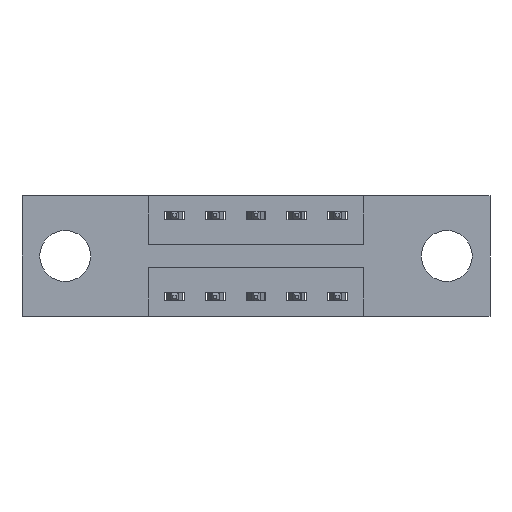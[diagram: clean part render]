
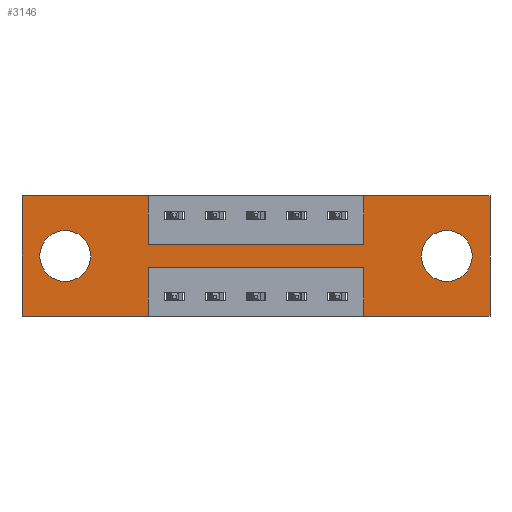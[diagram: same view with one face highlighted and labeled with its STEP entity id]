
A CAD part, front view. The second image highlights one B-rep face of the part: STEP entity #3146.
In plain terms, the highlighted planar face has unit normal (0, -1, 0).
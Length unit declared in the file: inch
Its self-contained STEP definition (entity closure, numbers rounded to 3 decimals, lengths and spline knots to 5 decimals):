
#69 = EDGE_CURVE ( 'NONE', #6793, #6067, #6084, .T. ) ;
#86 = EDGE_CURVE ( 'NONE', #6093, #6793, #6535, .T. ) ;
#127 = EDGE_CURVE ( 'NONE', #1687, #6093, #5450, .T. ) ;
#129 = CARTESIAN_POINT ( 'NONE',  ( 0.1325, 0., -0.185 ) ) ;
#203 = EDGE_CURVE ( 'NONE', #4125, #7672, #4257, .T. ) ;
#245 = CARTESIAN_POINT ( 'NONE',  ( 0.1325, 0., -0.263 ) ) ;
#272 = CARTESIAN_POINT ( 'NONE',  ( 0.3875, 0., 0. ) ) ;
#301 = VECTOR ( 'NONE', #5108, 39.37008 ) ;
#306 = DIRECTION ( 'NONE',  ( 0., 0., -1. ) ) ;
#368 = AXIS2_PLACEMENT_3D ( 'NONE', #5971, #5891, #1050 ) ;
#425 = CARTESIAN_POINT ( 'NONE',  ( 0.3875, 0., -0.37 ) ) ;
#450 = DIRECTION ( 'NONE',  ( 0., 0., -1. ) ) ;
#490 = CARTESIAN_POINT ( 'NONE',  ( 0.3875, 0., -0.15 ) ) ;
#520 = VECTOR ( 'NONE', #5414, 39.37008 ) ;
#553 = VERTEX_POINT ( 'NONE', #5676 ) ;
#614 = DIRECTION ( 'NONE',  ( 0., 0., 1. ) ) ;
#622 = CARTESIAN_POINT ( 'NONE',  ( 1.0475, 0., 0. ) ) ;
#652 = LINE ( 'NONE', #5789, #520 ) ;
#660 = EDGE_LOOP ( 'NONE', ( #7352, #1690, #7847, #6257, #4258, #1886, #1897, #4024, #5844, #7938, #4733, #712 ) ) ;
#696 = DIRECTION ( 'NONE',  ( 1., 0., 0. ) ) ;
#712 = ORIENTED_EDGE ( 'NONE', *, *, #5054, .F. ) ;
#835 = DIRECTION ( 'NONE',  ( 0., 0., -1. ) ) ;
#959 = DIRECTION ( 'NONE',  ( 0., 0., -1. ) ) ;
#968 = DIRECTION ( 'NONE',  ( 0., 1., 0. ) ) ;
#970 = CARTESIAN_POINT ( 'NONE',  ( 1.3025, 0., -0.185 ) ) ;
#979 = EDGE_CURVE ( 'NONE', #4657, #2655, #5480, .T. ) ;
#984 = EDGE_LOOP ( 'NONE', ( #4315, #3857 ) ) ;
#1050 = DIRECTION ( 'NONE',  ( 0., 0., -1. ) ) ;
#1095 = DIRECTION ( 'NONE',  ( 0., -1., 0. ) ) ;
#1530 = CIRCLE ( 'NONE', #3307, 0.078 ) ;
#1537 = VECTOR ( 'NONE', #450, 39.37008 ) ;
#1547 = LINE ( 'NONE', #425, #1537 ) ;
#1555 = EDGE_LOOP ( 'NONE', ( #2688, #7342 ) ) ;
#1558 = PLANE ( 'NONE',  #1777 ) ;
#1678 = VERTEX_POINT ( 'NONE', #3285 ) ;
#1687 = VERTEX_POINT ( 'NONE', #7633 ) ;
#1690 = ORIENTED_EDGE ( 'NONE', *, *, #7239, .F. ) ;
#1777 = AXIS2_PLACEMENT_3D ( 'NONE', #2217, #1095, #835 ) ;
#1886 = ORIENTED_EDGE ( 'NONE', *, *, #6462, .F. ) ;
#1897 = ORIENTED_EDGE ( 'NONE', *, *, #69, .F. ) ;
#1908 = VECTOR ( 'NONE', #5339, 39.37008 ) ;
#1909 = CARTESIAN_POINT ( 'NONE',  ( 1.3025, 0., -0.107 ) ) ;
#2067 = CARTESIAN_POINT ( 'NONE',  ( 1.435, 0., 0. ) ) ;
#2141 = VERTEX_POINT ( 'NONE', #8088 ) ;
#2177 = CARTESIAN_POINT ( 'NONE',  ( 1.435, 0., -0.37 ) ) ;
#2215 = EDGE_CURVE ( 'NONE', #2897, #1687, #2709, .T. ) ;
#2217 = CARTESIAN_POINT ( 'NONE',  ( 0., 0., -0.37 ) ) ;
#2349 = CARTESIAN_POINT ( 'NONE',  ( 0., 0., 0. ) ) ;
#2655 = VERTEX_POINT ( 'NONE', #2177 ) ;
#2688 = ORIENTED_EDGE ( 'NONE', *, *, #7082, .T. ) ;
#2709 = LINE ( 'NONE', #7521, #1908 ) ;
#2889 = EDGE_CURVE ( 'NONE', #2655, #2141, #5843, .T. ) ;
#2897 = VERTEX_POINT ( 'NONE', #2349 ) ;
#2913 = VERTEX_POINT ( 'NONE', #3804 ) ;
#2995 = CARTESIAN_POINT ( 'NONE',  ( 0., 0., 0. ) ) ;
#3004 = CARTESIAN_POINT ( 'NONE',  ( 1.435, 0., 0. ) ) ;
#3022 = CIRCLE ( 'NONE', #5811, 0.078 ) ;
#3045 = LINE ( 'NONE', #5154, #301 ) ;
#3075 = DIRECTION ( 'NONE',  ( 0., 0., 1. ) ) ;
#3105 = CARTESIAN_POINT ( 'NONE',  ( 1.0475, 0., -0.15 ) ) ;
#3142 = DIRECTION ( 'NONE',  ( -1., 0., 0. ) ) ;
#3146 = ADVANCED_FACE ( 'NONE', ( #5112, #7832, #4437 ), #1558, .T. ) ;
#3285 = CARTESIAN_POINT ( 'NONE',  ( 0.3875, 0., -0.22 ) ) ;
#3297 = EDGE_CURVE ( 'NONE', #4841, #2897, #7141, .T. ) ;
#3307 = AXIS2_PLACEMENT_3D ( 'NONE', #129, #8227, #8140 ) ;
#3403 = CARTESIAN_POINT ( 'NONE',  ( 0.1325, 0., -0.185 ) ) ;
#3646 = CARTESIAN_POINT ( 'NONE',  ( 0.1325, 0., -0.107 ) ) ;
#3804 = CARTESIAN_POINT ( 'NONE',  ( 1.0475, 0., -0.22 ) ) ;
#3857 = ORIENTED_EDGE ( 'NONE', *, *, #203, .T. ) ;
#3920 = CARTESIAN_POINT ( 'NONE',  ( 0.3875, 0., -0.37 ) ) ;
#4024 = ORIENTED_EDGE ( 'NONE', *, *, #86, .F. ) ;
#4125 = VERTEX_POINT ( 'NONE', #245 ) ;
#4225 = DIRECTION ( 'NONE',  ( 0., 0., -1. ) ) ;
#4257 = CIRCLE ( 'NONE', #4466, 0.078 ) ;
#4258 = ORIENTED_EDGE ( 'NONE', *, *, #979, .F. ) ;
#4315 = ORIENTED_EDGE ( 'NONE', *, *, #7189, .T. ) ;
#4417 = VECTOR ( 'NONE', #3142, 39.37008 ) ;
#4437 = FACE_OUTER_BOUND ( 'NONE', #660, .T. ) ;
#4466 = AXIS2_PLACEMENT_3D ( 'NONE', #3403, #8249, #5424 ) ;
#4657 = VERTEX_POINT ( 'NONE', #3004 ) ;
#4733 = ORIENTED_EDGE ( 'NONE', *, *, #3297, .F. ) ;
#4841 = VERTEX_POINT ( 'NONE', #7290 ) ;
#4845 = EDGE_CURVE ( 'NONE', #553, #5308, #6419, .T. ) ;
#5046 = VECTOR ( 'NONE', #306, 39.37008 ) ;
#5054 = EDGE_CURVE ( 'NONE', #5716, #4841, #6708, .T. ) ;
#5108 = DIRECTION ( 'NONE',  ( 1., 0., 0. ) ) ;
#5112 = FACE_BOUND ( 'NONE', #1555, .T. ) ;
#5154 = CARTESIAN_POINT ( 'NONE',  ( 0., 0., 0. ) ) ;
#5299 = VECTOR ( 'NONE', #4225, 39.37008 ) ;
#5308 = VERTEX_POINT ( 'NONE', #1909 ) ;
#5339 = DIRECTION ( 'NONE',  ( 1., 0., 0. ) ) ;
#5369 = VECTOR ( 'NONE', #8234, 39.37008 ) ;
#5413 = LINE ( 'NONE', #8226, #5369 ) ;
#5414 = DIRECTION ( 'NONE',  ( -1., 0., 0. ) ) ;
#5424 = DIRECTION ( 'NONE',  ( 0., 0., 1. ) ) ;
#5450 = LINE ( 'NONE', #272, #5046 ) ;
#5480 = LINE ( 'NONE', #2067, #5299 ) ;
#5541 = DIRECTION ( 'NONE',  ( -1., 0., 0. ) ) ;
#5676 = CARTESIAN_POINT ( 'NONE',  ( 1.3025, 0., -0.263 ) ) ;
#5716 = VERTEX_POINT ( 'NONE', #3920 ) ;
#5789 = CARTESIAN_POINT ( 'NONE',  ( 0.3875, 0., -0.22 ) ) ;
#5811 = AXIS2_PLACEMENT_3D ( 'NONE', #970, #968, #959 ) ;
#5843 = LINE ( 'NONE', #6391, #4417 ) ;
#5844 = ORIENTED_EDGE ( 'NONE', *, *, #127, .F. ) ;
#5891 = DIRECTION ( 'NONE',  ( 0., 1., 0. ) ) ;
#5971 = CARTESIAN_POINT ( 'NONE',  ( 1.3025, 0., -0.185 ) ) ;
#6067 = VERTEX_POINT ( 'NONE', #7946 ) ;
#6084 = LINE ( 'NONE', #622, #6367 ) ;
#6087 = VECTOR ( 'NONE', #3075, 39.37008 ) ;
#6093 = VERTEX_POINT ( 'NONE', #7624 ) ;
#6178 = VECTOR ( 'NONE', #696, 39.37008 ) ;
#6257 = ORIENTED_EDGE ( 'NONE', *, *, #2889, .F. ) ;
#6284 = CARTESIAN_POINT ( 'NONE',  ( 0., 0., -0.37 ) ) ;
#6367 = VECTOR ( 'NONE', #614, 39.37008 ) ;
#6391 = CARTESIAN_POINT ( 'NONE',  ( 0., 0., -0.37 ) ) ;
#6419 = CIRCLE ( 'NONE', #368, 0.078 ) ;
#6462 = EDGE_CURVE ( 'NONE', #6067, #4657, #3045, .T. ) ;
#6535 = LINE ( 'NONE', #490, #6178 ) ;
#6685 = VECTOR ( 'NONE', #5541, 39.37008 ) ;
#6708 = LINE ( 'NONE', #6284, #6685 ) ;
#6793 = VERTEX_POINT ( 'NONE', #3105 ) ;
#7082 = EDGE_CURVE ( 'NONE', #5308, #553, #3022, .T. ) ;
#7140 = EDGE_CURVE ( 'NONE', #1678, #5716, #1547, .T. ) ;
#7141 = LINE ( 'NONE', #2995, #6087 ) ;
#7189 = EDGE_CURVE ( 'NONE', #7672, #4125, #1530, .T. ) ;
#7239 = EDGE_CURVE ( 'NONE', #2913, #1678, #652, .T. ) ;
#7290 = CARTESIAN_POINT ( 'NONE',  ( 0., 0., -0.37 ) ) ;
#7342 = ORIENTED_EDGE ( 'NONE', *, *, #4845, .T. ) ;
#7352 = ORIENTED_EDGE ( 'NONE', *, *, #7140, .F. ) ;
#7521 = CARTESIAN_POINT ( 'NONE',  ( 0., 0., 0. ) ) ;
#7624 = CARTESIAN_POINT ( 'NONE',  ( 0.3875, 0., -0.15 ) ) ;
#7633 = CARTESIAN_POINT ( 'NONE',  ( 0.3875, 0., 0. ) ) ;
#7672 = VERTEX_POINT ( 'NONE', #3646 ) ;
#7832 = FACE_BOUND ( 'NONE', #984, .T. ) ;
#7847 = ORIENTED_EDGE ( 'NONE', *, *, #7892, .F. ) ;
#7892 = EDGE_CURVE ( 'NONE', #2141, #2913, #5413, .T. ) ;
#7938 = ORIENTED_EDGE ( 'NONE', *, *, #2215, .F. ) ;
#7946 = CARTESIAN_POINT ( 'NONE',  ( 1.0475, 0., 0. ) ) ;
#8088 = CARTESIAN_POINT ( 'NONE',  ( 1.0475, 0., -0.37 ) ) ;
#8140 = DIRECTION ( 'NONE',  ( 0., 0., 1. ) ) ;
#8226 = CARTESIAN_POINT ( 'NONE',  ( 1.0475, 0., -0.37 ) ) ;
#8227 = DIRECTION ( 'NONE',  ( 0., 1., 0. ) ) ;
#8234 = DIRECTION ( 'NONE',  ( 0., 0., 1. ) ) ;
#8249 = DIRECTION ( 'NONE',  ( 0., 1., 0. ) ) ;
